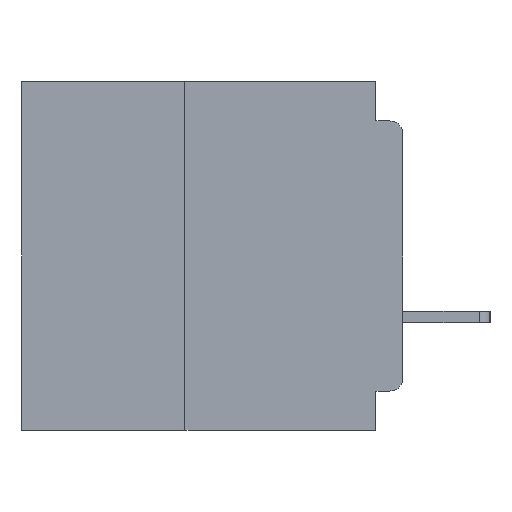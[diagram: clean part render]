
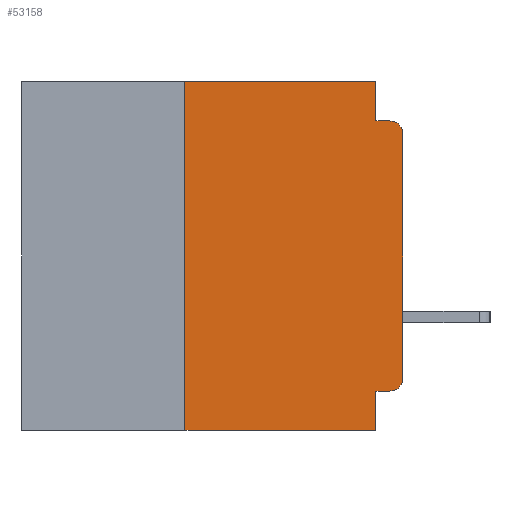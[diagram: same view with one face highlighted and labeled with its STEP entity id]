
A CAD part, left-side view. The second image highlights one B-rep face of the part: STEP entity #53158.
In plain terms, the highlighted planar face has unit normal (-1, 0, 0).
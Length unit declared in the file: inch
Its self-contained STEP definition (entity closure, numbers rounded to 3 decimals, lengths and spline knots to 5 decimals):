
#348 = CARTESIAN_POINT ( 'NONE',  ( 0., 0.437, 0. ) ) ;
#1270 = LINE ( 'NONE', #5062, #38518 ) ;
#3846 = LINE ( 'NONE', #34312, #13371 ) ;
#4949 = DIRECTION ( 'NONE',  ( 0., 0., -1. ) ) ;
#5062 = CARTESIAN_POINT ( 'NONE',  ( 0., 0., -0.355 ) ) ;
#5129 = DIRECTION ( 'NONE',  ( 0., -1., 0. ) ) ;
#5549 = CARTESIAN_POINT ( 'NONE',  ( 0., 0.25, -0.4 ) ) ;
#10286 = DIRECTION ( 'NONE',  ( 0., 0., 1. ) ) ;
#10511 = CIRCLE ( 'NONE', #13635, 0.015 ) ;
#11698 = CARTESIAN_POINT ( 'NONE',  ( 0., 0.015, -0.34 ) ) ;
#11994 = VERTEX_POINT ( 'NONE', #55119 ) ;
#12647 = VERTEX_POINT ( 'NONE', #40260 ) ;
#13371 = VECTOR ( 'NONE', #38966, 39.37008 ) ;
#13526 = VECTOR ( 'NONE', #5129, 39.37008 ) ;
#13635 = AXIS2_PLACEMENT_3D ( 'NONE', #11698, #44177, #16384 ) ;
#14069 = EDGE_CURVE ( 'NONE', #51444, #31128, #1270, .T. ) ;
#15142 = CARTESIAN_POINT ( 'NONE',  ( 0., 0., 0. ) ) ;
#15898 = EDGE_CURVE ( 'NONE', #30080, #11994, #20099, .T. ) ;
#16384 = DIRECTION ( 'NONE',  ( 0., 0., -1. ) ) ;
#16480 = CARTESIAN_POINT ( 'NONE',  ( 0., 0.015, -0.355 ) ) ;
#17659 = EDGE_CURVE ( 'NONE', #20954, #45282, #20723, .T. ) ;
#17705 = EDGE_CURVE ( 'NONE', #34818, #30080, #45411, .T. ) ;
#18125 = PLANE ( 'NONE',  #25268 ) ;
#18887 = ORIENTED_EDGE ( 'NONE', *, *, #53643, .F. ) ;
#20099 = CIRCLE ( 'NONE', #36612, 0.015 ) ;
#20723 = LINE ( 'NONE', #5549, #56197 ) ;
#20948 = ORIENTED_EDGE ( 'NONE', *, *, #15898, .T. ) ;
#20954 = VERTEX_POINT ( 'NONE', #26591 ) ;
#21339 = LINE ( 'NONE', #29319, #56806 ) ;
#21387 = ORIENTED_EDGE ( 'NONE', *, *, #17659, .F. ) ;
#21573 = ORIENTED_EDGE ( 'NONE', *, *, #17705, .T. ) ;
#22096 = CARTESIAN_POINT ( 'NONE',  ( 0., 0., -0.34 ) ) ;
#22460 = VECTOR ( 'NONE', #53881, 39.37008 ) ;
#22828 = DIRECTION ( 'NONE',  ( 1., 0., 0. ) ) ;
#23697 = VECTOR ( 'NONE', #4949, 39.37008 ) ;
#25192 = LINE ( 'NONE', #51233, #23697 ) ;
#25247 = EDGE_CURVE ( 'NONE', #25389, #11994, #3846, .T. ) ;
#25268 = AXIS2_PLACEMENT_3D ( 'NONE', #50508, #22828, #55166 ) ;
#25389 = VERTEX_POINT ( 'NONE', #35319 ) ;
#25424 = DIRECTION ( 'NONE',  ( -1., 0., 0. ) ) ;
#25799 = ORIENTED_EDGE ( 'NONE', *, *, #25247, .F. ) ;
#26458 = EDGE_CURVE ( 'NONE', #20954, #38482, #21339, .T. ) ;
#26591 = CARTESIAN_POINT ( 'NONE',  ( 0., 0.25, -0.4 ) ) ;
#29319 = CARTESIAN_POINT ( 'NONE',  ( 0., 0.437, -0.4 ) ) ;
#29678 = CARTESIAN_POINT ( 'NONE',  ( 0., 0., -0.06 ) ) ;
#30080 = VERTEX_POINT ( 'NONE', #29678 ) ;
#31128 = VERTEX_POINT ( 'NONE', #41886 ) ;
#33019 = DIRECTION ( 'NONE',  ( 0., 1., 0. ) ) ;
#34312 = CARTESIAN_POINT ( 'NONE',  ( 0., 0., -0.045 ) ) ;
#34818 = VERTEX_POINT ( 'NONE', #22096 ) ;
#35319 = CARTESIAN_POINT ( 'NONE',  ( 0., 0.031, -0.045 ) ) ;
#36217 = CARTESIAN_POINT ( 'NONE',  ( 0., 0.25, 0. ) ) ;
#36612 = AXIS2_PLACEMENT_3D ( 'NONE', #53036, #25424, #57714 ) ;
#37765 = FACE_OUTER_BOUND ( 'NONE', #50786, .T. ) ;
#38122 = ORIENTED_EDGE ( 'NONE', *, *, #55591, .T. ) ;
#38482 = VERTEX_POINT ( 'NONE', #49635 ) ;
#38518 = VECTOR ( 'NONE', #33019, 39.37008 ) ;
#38774 = ORIENTED_EDGE ( 'NONE', *, *, #48286, .F. ) ;
#38966 = DIRECTION ( 'NONE',  ( 0., -1., 0. ) ) ;
#39704 = LINE ( 'NONE', #348, #13526 ) ;
#40260 = CARTESIAN_POINT ( 'NONE',  ( 0., 0.031, 0. ) ) ;
#41886 = CARTESIAN_POINT ( 'NONE',  ( 0., 0.031, -0.355 ) ) ;
#44177 = DIRECTION ( 'NONE',  ( -1., 0., 0. ) ) ;
#44443 = ORIENTED_EDGE ( 'NONE', *, *, #55310, .F. ) ;
#45282 = VERTEX_POINT ( 'NONE', #36217 ) ;
#45411 = LINE ( 'NONE', #15142, #54754 ) ;
#48286 = EDGE_CURVE ( 'NONE', #45282, #12647, #39704, .T. ) ;
#49242 = CARTESIAN_POINT ( 'NONE',  ( 0., 0.031, -0.4 ) ) ;
#49635 = CARTESIAN_POINT ( 'NONE',  ( 0., 0.031, -0.4 ) ) ;
#50508 = CARTESIAN_POINT ( 'NONE',  ( 0., 0.437, 0. ) ) ;
#50786 = EDGE_LOOP ( 'NONE', ( #21573, #20948, #25799, #44443, #38774, #21387, #57935, #18887, #52281, #38122 ) ) ;
#51233 = CARTESIAN_POINT ( 'NONE',  ( 0., 0.031, 0. ) ) ;
#51444 = VERTEX_POINT ( 'NONE', #16480 ) ;
#52217 = DIRECTION ( 'NONE',  ( 0., 0., 1. ) ) ;
#52281 = ORIENTED_EDGE ( 'NONE', *, *, #14069, .F. ) ;
#52288 = DIRECTION ( 'NONE',  ( 0., -1., 0. ) ) ;
#53036 = CARTESIAN_POINT ( 'NONE',  ( 0., 0.015, -0.06 ) ) ;
#53158 = ADVANCED_FACE ( 'NONE', ( #37765 ), #18125, .F. ) ;
#53643 = EDGE_CURVE ( 'NONE', #31128, #38482, #59382, .T. ) ;
#53881 = DIRECTION ( 'NONE',  ( 0., 0., -1. ) ) ;
#54754 = VECTOR ( 'NONE', #52217, 39.37008 ) ;
#55119 = CARTESIAN_POINT ( 'NONE',  ( 0., 0.015, -0.045 ) ) ;
#55166 = DIRECTION ( 'NONE',  ( 0., 0., -1. ) ) ;
#55310 = EDGE_CURVE ( 'NONE', #12647, #25389, #25192, .T. ) ;
#55591 = EDGE_CURVE ( 'NONE', #51444, #34818, #10511, .T. ) ;
#56197 = VECTOR ( 'NONE', #10286, 39.37008 ) ;
#56806 = VECTOR ( 'NONE', #52288, 39.37008 ) ;
#57714 = DIRECTION ( 'NONE',  ( 0., 0., -1. ) ) ;
#57935 = ORIENTED_EDGE ( 'NONE', *, *, #26458, .T. ) ;
#59382 = LINE ( 'NONE', #49242, #22460 ) ;
